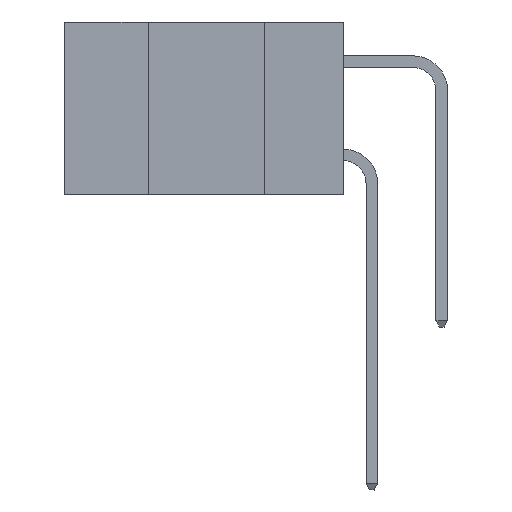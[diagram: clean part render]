
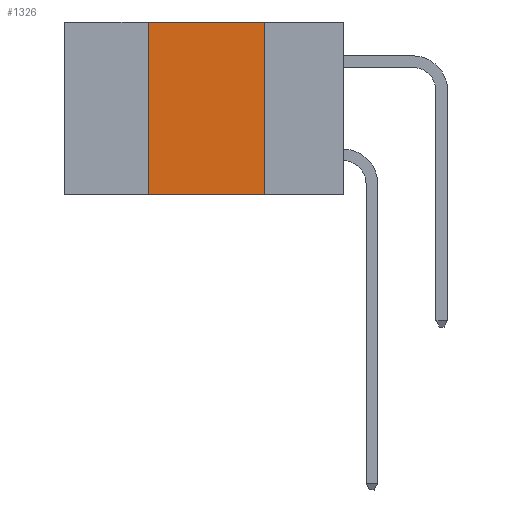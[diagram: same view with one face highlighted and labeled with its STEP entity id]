
A CAD part, left-side view. The second image highlights one B-rep face of the part: STEP entity #1326.
In plain terms, the highlighted planar face has unit normal (-1, 0, 0).
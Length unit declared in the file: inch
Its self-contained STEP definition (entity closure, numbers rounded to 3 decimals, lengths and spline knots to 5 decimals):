
#330 = LINE ( 'NONE', #3754, #1507 ) ;
#343 = DIRECTION ( 'NONE',  ( 0., 0., -1. ) ) ;
#653 = CARTESIAN_POINT ( 'NONE',  ( 0., 0.42, -0.37 ) ) ;
#939 = CARTESIAN_POINT ( 'NONE',  ( 0., 0.42, -0.37 ) ) ;
#1326 = ADVANCED_FACE ( 'NONE', ( #3706 ), #7340, .F. ) ;
#1418 = LINE ( 'NONE', #8579, #2719 ) ;
#1507 = VECTOR ( 'NONE', #6661, 39.37008 ) ;
#2054 = CARTESIAN_POINT ( 'NONE',  ( 0., 0.6, 0. ) ) ;
#2719 = VECTOR ( 'NONE', #343, 39.37008 ) ;
#2855 = AXIS2_PLACEMENT_3D ( 'NONE', #2054, #4637, #8378 ) ;
#3157 = EDGE_LOOP ( 'NONE', ( #11557, #5286, #8407, #8767 ) ) ;
#3386 = LINE ( 'NONE', #653, #8676 ) ;
#3472 = CARTESIAN_POINT ( 'NONE',  ( 0., 0.17, 0. ) ) ;
#3706 = FACE_OUTER_BOUND ( 'NONE', #3157, .T. ) ;
#3744 = CARTESIAN_POINT ( 'NONE',  ( 0., 0.17, -0.37 ) ) ;
#3754 = CARTESIAN_POINT ( 'NONE',  ( 0., 0.6, -0.37 ) ) ;
#4003 = EDGE_CURVE ( 'NONE', #11323, #8284, #3386, .T. ) ;
#4175 = CARTESIAN_POINT ( 'NONE',  ( 0., 0.6, 0. ) ) ;
#4637 = DIRECTION ( 'NONE',  ( 1., 0., 0. ) ) ;
#4704 = EDGE_CURVE ( 'NONE', #11323, #5214, #330, .T. ) ;
#5214 = VERTEX_POINT ( 'NONE', #3744 ) ;
#5280 = DIRECTION ( 'NONE',  ( 0., 0., 1. ) ) ;
#5286 = ORIENTED_EDGE ( 'NONE', *, *, #9133, .F. ) ;
#6649 = LINE ( 'NONE', #4175, #8158 ) ;
#6661 = DIRECTION ( 'NONE',  ( 0., -1., 0. ) ) ;
#7340 = PLANE ( 'NONE',  #2855 ) ;
#7943 = VERTEX_POINT ( 'NONE', #3472 ) ;
#8158 = VECTOR ( 'NONE', #8488, 39.37008 ) ;
#8284 = VERTEX_POINT ( 'NONE', #11095 ) ;
#8378 = DIRECTION ( 'NONE',  ( 0., 0., -1. ) ) ;
#8407 = ORIENTED_EDGE ( 'NONE', *, *, #4003, .F. ) ;
#8488 = DIRECTION ( 'NONE',  ( 0., -1., 0. ) ) ;
#8579 = CARTESIAN_POINT ( 'NONE',  ( 0., 0.17, -0.37 ) ) ;
#8676 = VECTOR ( 'NONE', #5280, 39.37008 ) ;
#8767 = ORIENTED_EDGE ( 'NONE', *, *, #4704, .T. ) ;
#9133 = EDGE_CURVE ( 'NONE', #8284, #7943, #6649, .T. ) ;
#10079 = EDGE_CURVE ( 'NONE', #7943, #5214, #1418, .T. ) ;
#11095 = CARTESIAN_POINT ( 'NONE',  ( 0., 0.42, 0. ) ) ;
#11323 = VERTEX_POINT ( 'NONE', #939 ) ;
#11557 = ORIENTED_EDGE ( 'NONE', *, *, #10079, .F. ) ;
